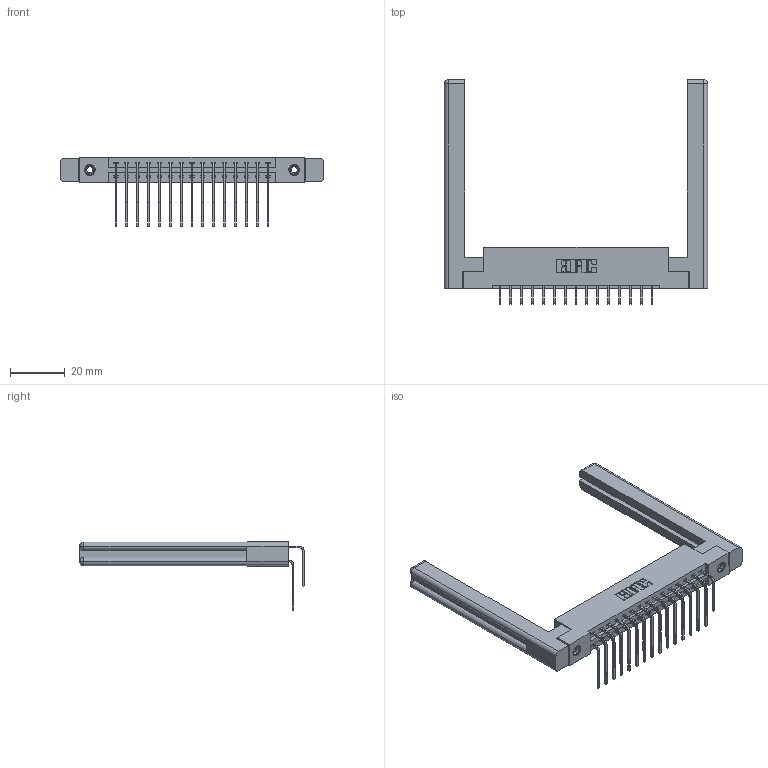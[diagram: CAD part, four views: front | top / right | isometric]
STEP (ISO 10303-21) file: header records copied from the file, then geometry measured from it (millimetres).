
FILE_DESCRIPTION (( 'STEP AP203' ), '1' );
FILE_NAME ('337-030-559-258.STEP', '2019-10-08T19:03:08', ( '' ), ( '' ), 'SwSTEP 2.0', 'SolidWorks 2016', '' );
FILE_SCHEMA (( 'CONFIG_CONTROL_DESIGN' ));
Length unit declared in the file: inch
Products named in the file (6): 345-292-001_558 559 Tail - 1; 307-220-058; 345-250-001_345-250-001-102; 337 Part_Flush Mounting Lugs - 0.156 Dia-TI; 337-030-559-258; 345-292-001_559 Tail - 2
Assembly tree (35 placements, depth 2):
  337-030-559-258
    337 Part_Flush Mounting Lugs - 0.156 Dia-TI
    345-292-001_558 559 Tail - 1  x15
    345-292-001_559 Tail - 2  x15
    345-250-001_345-250-001-102  x2
    307-220-058  x2
Bounding box: 96.06 x 81.98 x 25.53 mm (x, y, z)
Volume: 17079.9 mm3; surface area: 16887.9 mm2
Topology: 35 solids, 35 shells, 1936 faces, 5675 edges, 3730 vertices
Faces by surface type: plane 1354, cylinder 558, cone 12, torus 12
Entity records: 19540 total; most frequent: CARTESIAN_POINT 3368, ORIENTED_EDGE 3192, DIRECTION 2912, EDGE_CURVE 1596, VECTOR 1380, LINE 1380, VERTEX_POINT 1054, AXIS2_PLACEMENT_3D 766
